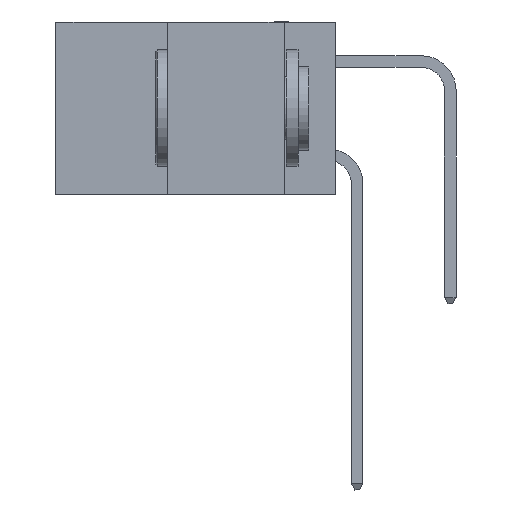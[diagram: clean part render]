
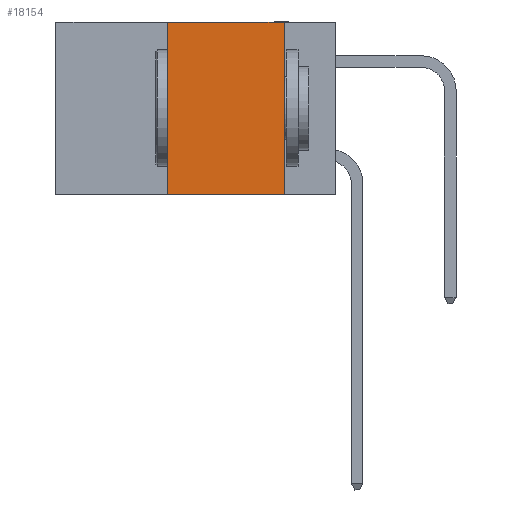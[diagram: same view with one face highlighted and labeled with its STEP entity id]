
A CAD part, left-side view. The second image highlights one B-rep face of the part: STEP entity #18154.
In plain terms, the highlighted planar face has unit normal (-1, 0, 0).
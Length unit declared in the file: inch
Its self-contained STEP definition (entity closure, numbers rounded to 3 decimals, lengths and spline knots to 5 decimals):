
#5 = DIRECTION ( 'NONE',  ( 0., -1., 0. ) ) ;
#293 = EDGE_CURVE ( 'NONE', #31858, #13821, #28280, .T. ) ;
#933 = LINE ( 'NONE', #14786, #33940 ) ;
#1581 = CARTESIAN_POINT ( 'NONE',  ( 0., 0.11, -0.37 ) ) ;
#2180 = ORIENTED_EDGE ( 'NONE', *, *, #3224, .F. ) ;
#2183 = ORIENTED_EDGE ( 'NONE', *, *, #2282, .F. ) ;
#2282 = EDGE_CURVE ( 'NONE', #11870, #31858, #32631, .T. ) ;
#3224 = EDGE_CURVE ( 'NONE', #22935, #11870, #933, .T. ) ;
#4526 = EDGE_LOOP ( 'NONE', ( #18011, #2183, #2180, #6405 ) ) ;
#6405 = ORIENTED_EDGE ( 'NONE', *, *, #23623, .T. ) ;
#6710 = DIRECTION ( 'NONE',  ( 0., 0., -1. ) ) ;
#8255 = VECTOR ( 'NONE', #5, 39.37008 ) ;
#10127 = CARTESIAN_POINT ( 'NONE',  ( 0., 0.11, 0. ) ) ;
#11084 = VECTOR ( 'NONE', #17620, 39.37008 ) ;
#11870 = VERTEX_POINT ( 'NONE', #33586 ) ;
#13426 = DIRECTION ( 'NONE',  ( 1., 0., 0. ) ) ;
#13821 = VERTEX_POINT ( 'NONE', #1581 ) ;
#14225 = CARTESIAN_POINT ( 'NONE',  ( 0., 0.36, -0.37 ) ) ;
#14786 = CARTESIAN_POINT ( 'NONE',  ( 0., 0.36, 0. ) ) ;
#17620 = DIRECTION ( 'NONE',  ( 0., 0., -1. ) ) ;
#18011 = ORIENTED_EDGE ( 'NONE', *, *, #293, .F. ) ;
#18154 = ADVANCED_FACE ( 'NONE', ( #20602 ), #25507, .F. ) ;
#20390 = CARTESIAN_POINT ( 'NONE',  ( 0., 0.11, 0. ) ) ;
#20602 = FACE_OUTER_BOUND ( 'NONE', #4526, .T. ) ;
#20785 = AXIS2_PLACEMENT_3D ( 'NONE', #27810, #13426, #6710 ) ;
#21293 = CARTESIAN_POINT ( 'NONE',  ( 0., 0.6, -0.37 ) ) ;
#21802 = DIRECTION ( 'NONE',  ( 0., -1., 0. ) ) ;
#22935 = VERTEX_POINT ( 'NONE', #14225 ) ;
#22947 = CARTESIAN_POINT ( 'NONE',  ( 0., 0.6, 0. ) ) ;
#23623 = EDGE_CURVE ( 'NONE', #22935, #13821, #24253, .T. ) ;
#24253 = LINE ( 'NONE', #21293, #28829 ) ;
#25507 = PLANE ( 'NONE',  #20785 ) ;
#27810 = CARTESIAN_POINT ( 'NONE',  ( 0., 0.6, 0. ) ) ;
#28280 = LINE ( 'NONE', #10127, #11084 ) ;
#28829 = VECTOR ( 'NONE', #21802, 39.37008 ) ;
#31858 = VERTEX_POINT ( 'NONE', #20390 ) ;
#32631 = LINE ( 'NONE', #22947, #8255 ) ;
#33586 = CARTESIAN_POINT ( 'NONE',  ( 0., 0.36, 0. ) ) ;
#33940 = VECTOR ( 'NONE', #35273, 39.37008 ) ;
#35273 = DIRECTION ( 'NONE',  ( 0., 0., 1. ) ) ;
